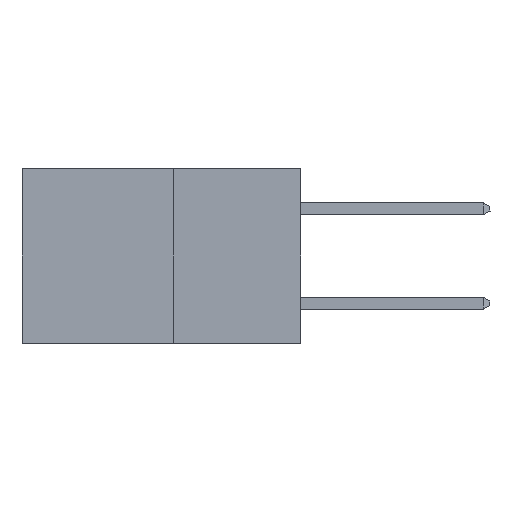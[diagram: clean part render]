
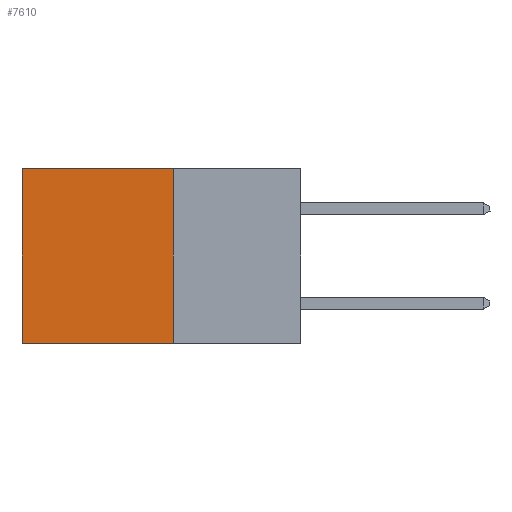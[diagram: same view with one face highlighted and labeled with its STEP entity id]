
A CAD part, left-side view. The second image highlights one B-rep face of the part: STEP entity #7610.
In plain terms, the highlighted planar face has unit normal (-1, 0, 0).
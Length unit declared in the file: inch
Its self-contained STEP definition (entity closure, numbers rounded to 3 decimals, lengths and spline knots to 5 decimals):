
#449 = EDGE_LOOP ( 'NONE', ( #8101, #3111, #10595, #5473 ) ) ;
#532 = EDGE_CURVE ( 'NONE', #3115, #1115, #5556, .T. ) ;
#550 = VECTOR ( 'NONE', #7571, 39.37008 ) ;
#1115 = VERTEX_POINT ( 'NONE', #7664 ) ;
#2056 = CARTESIAN_POINT ( 'NONE',  ( 0.277, 0.59, 0. ) ) ;
#2100 = DIRECTION ( 'NONE',  ( 0., 1., 0. ) ) ;
#2148 = DIRECTION ( 'NONE',  ( 0., 0., -1. ) ) ;
#3045 = LINE ( 'NONE', #10662, #7299 ) ;
#3111 = ORIENTED_EDGE ( 'NONE', *, *, #532, .F. ) ;
#3115 = VERTEX_POINT ( 'NONE', #7020 ) ;
#3808 = EDGE_CURVE ( 'NONE', #8387, #1115, #3045, .T. ) ;
#4423 = LINE ( 'NONE', #6885, #8536 ) ;
#4754 = CARTESIAN_POINT ( 'NONE',  ( 0.277, 0.27, 0. ) ) ;
#5473 = ORIENTED_EDGE ( 'NONE', *, *, #10758, .T. ) ;
#5556 = LINE ( 'NONE', #7483, #550 ) ;
#6077 = EDGE_CURVE ( 'NONE', #9675, #3115, #4423, .T. ) ;
#6453 = CARTESIAN_POINT ( 'NONE',  ( 0.277, 0.27, -0.37 ) ) ;
#6885 = CARTESIAN_POINT ( 'NONE',  ( 0.277, 0.27, -0.37 ) ) ;
#6898 = DIRECTION ( 'NONE',  ( 0., 0., -1. ) ) ;
#6927 = CARTESIAN_POINT ( 'NONE',  ( 0.277, 0.27, 0. ) ) ;
#6978 = DIRECTION ( 'NONE',  ( 0., 0., -1. ) ) ;
#7020 = CARTESIAN_POINT ( 'NONE',  ( 0.277, 0.27, -0.37 ) ) ;
#7285 = DIRECTION ( 'NONE',  ( 1., 0., 0. ) ) ;
#7299 = VECTOR ( 'NONE', #6978, 39.37008 ) ;
#7483 = CARTESIAN_POINT ( 'NONE',  ( 0.277, 0.27, -0.37 ) ) ;
#7515 = FACE_OUTER_BOUND ( 'NONE', #449, .T. ) ;
#7571 = DIRECTION ( 'NONE',  ( 0., 1., 0. ) ) ;
#7610 = ADVANCED_FACE ( 'NONE', ( #7515 ), #10469, .F. ) ;
#7664 = CARTESIAN_POINT ( 'NONE',  ( 0.277, 0.59, -0.37 ) ) ;
#8101 = ORIENTED_EDGE ( 'NONE', *, *, #3808, .T. ) ;
#8387 = VERTEX_POINT ( 'NONE', #2056 ) ;
#8536 = VECTOR ( 'NONE', #6898, 39.37008 ) ;
#8893 = AXIS2_PLACEMENT_3D ( 'NONE', #6453, #7285, #2148 ) ;
#9675 = VERTEX_POINT ( 'NONE', #6927 ) ;
#10452 = VECTOR ( 'NONE', #2100, 39.37008 ) ;
#10469 = PLANE ( 'NONE',  #8893 ) ;
#10595 = ORIENTED_EDGE ( 'NONE', *, *, #6077, .F. ) ;
#10662 = CARTESIAN_POINT ( 'NONE',  ( 0.277, 0.59, -0.37 ) ) ;
#10698 = LINE ( 'NONE', #4754, #10452 ) ;
#10758 = EDGE_CURVE ( 'NONE', #9675, #8387, #10698, .T. ) ;
